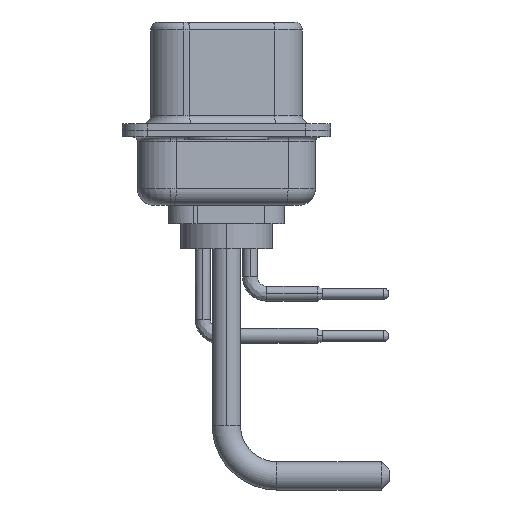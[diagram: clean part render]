
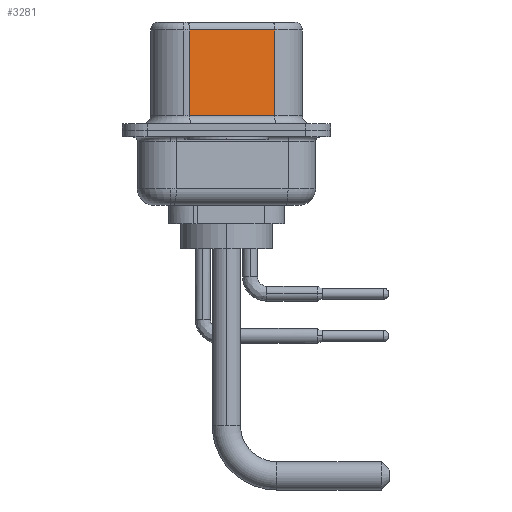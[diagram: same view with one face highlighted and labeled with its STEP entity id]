
A CAD part, left-side view. The second image highlights one B-rep face of the part: STEP entity #3281.
In plain terms, the highlighted planar face has unit normal (-0.985, -0.174, 0).
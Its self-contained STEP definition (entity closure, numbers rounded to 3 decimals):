
#1091 = CARTESIAN_POINT ( 'NONE',  ( 4.58, -2.897, 6.52 ) ) ;
#2255 = EDGE_CURVE ( 'NONE', #8569, #5104, #12261, .T. ) ;
#3281 = ADVANCED_FACE ( 'NONE', ( #11651 ), #23305, .F. ) ;
#4006 = VERTEX_POINT ( 'NONE', #11061 ) ;
#5104 = VERTEX_POINT ( 'NONE', #10159 ) ;
#5123 = ORIENTED_EDGE ( 'NONE', *, *, #2255, .F. ) ;
#5646 = CARTESIAN_POINT ( 'NONE',  ( 4.58, -2.897, 0.9 ) ) ;
#6040 = DIRECTION ( 'NONE',  ( -0.174, 0.985, 0. ) ) ;
#6318 = DIRECTION ( 'NONE',  ( -0.174, 0.985, 0. ) ) ;
#6909 = ORIENTED_EDGE ( 'NONE', *, *, #14113, .T. ) ;
#8569 = VERTEX_POINT ( 'NONE', #20963 ) ;
#10159 = CARTESIAN_POINT ( 'NONE',  ( 4.58, -2.897, 0.9 ) ) ;
#11061 = CARTESIAN_POINT ( 'NONE',  ( 3.68, 2.203, 6.02 ) ) ;
#11195 = DIRECTION ( 'NONE',  ( 0., 0., -1. ) ) ;
#11651 = FACE_OUTER_BOUND ( 'NONE', #25418, .T. ) ;
#11809 = LINE ( 'NONE', #19998, #21921 ) ;
#12261 = LINE ( 'NONE', #14365, #12390 ) ;
#12390 = VECTOR ( 'NONE', #22432, 1000. ) ;
#14113 = EDGE_CURVE ( 'NONE', #17876, #5104, #15712, .T. ) ;
#14365 = CARTESIAN_POINT ( 'NONE',  ( 4.58, -2.897, 6.52 ) ) ;
#14382 = EDGE_CURVE ( 'NONE', #8569, #4006, #16507, .T. ) ;
#15712 = LINE ( 'NONE', #5646, #19378 ) ;
#16507 = LINE ( 'NONE', #20616, #17919 ) ;
#16848 = ORIENTED_EDGE ( 'NONE', *, *, #19341, .T. ) ;
#17370 = CARTESIAN_POINT ( 'NONE',  ( 3.68, 2.203, 0.9 ) ) ;
#17876 = VERTEX_POINT ( 'NONE', #17370 ) ;
#17919 = VECTOR ( 'NONE', #6318, 1000. ) ;
#19341 = EDGE_CURVE ( 'NONE', #4006, #17876, #11809, .T. ) ;
#19378 = VECTOR ( 'NONE', #25616, 1000. ) ;
#19733 = DIRECTION ( 'NONE',  ( 0.985, 0.174, 0. ) ) ;
#19998 = CARTESIAN_POINT ( 'NONE',  ( 3.68, 2.203, 6.52 ) ) ;
#20616 = CARTESIAN_POINT ( 'NONE',  ( 4.58, -2.897, 6.02 ) ) ;
#20963 = CARTESIAN_POINT ( 'NONE',  ( 4.58, -2.897, 6.02 ) ) ;
#21921 = VECTOR ( 'NONE', #11195, 1000. ) ;
#22079 = AXIS2_PLACEMENT_3D ( 'NONE', #1091, #19733, #6040 ) ;
#22123 = ORIENTED_EDGE ( 'NONE', *, *, #14382, .T. ) ;
#22432 = DIRECTION ( 'NONE',  ( 0., 0., -1. ) ) ;
#23305 = PLANE ( 'NONE',  #22079 ) ;
#25418 = EDGE_LOOP ( 'NONE', ( #5123, #22123, #16848, #6909 ) ) ;
#25616 = DIRECTION ( 'NONE',  ( 0.174, -0.985, 0. ) ) ;
